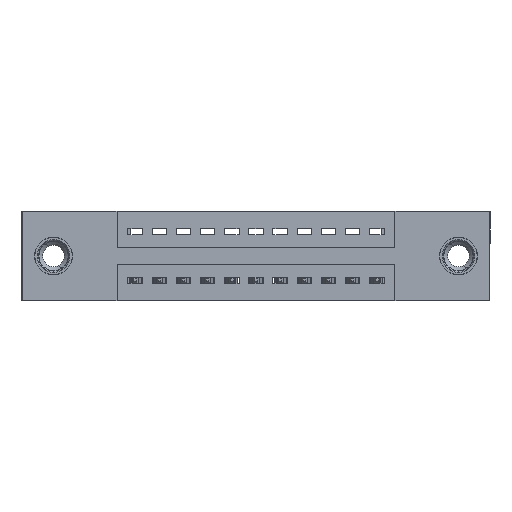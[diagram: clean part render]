
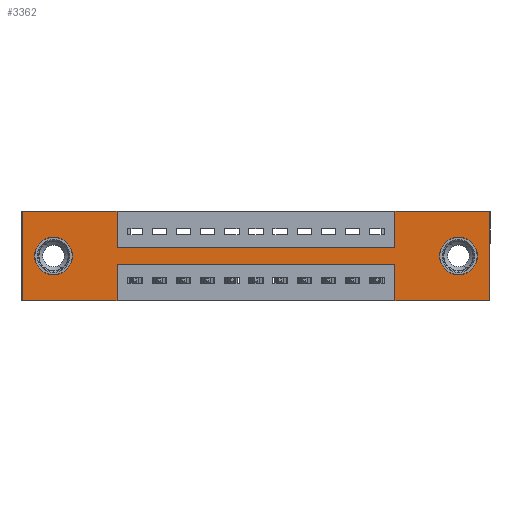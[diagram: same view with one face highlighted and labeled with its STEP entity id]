
A CAD part, front view. The second image highlights one B-rep face of the part: STEP entity #3362.
In plain terms, the highlighted planar face has unit normal (0, -1, 0).
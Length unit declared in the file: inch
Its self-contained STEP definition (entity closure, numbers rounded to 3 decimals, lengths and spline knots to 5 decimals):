
#35 = CARTESIAN_POINT ( 'NONE',  ( 0.3925, 0., -0.22 ) ) ;
#104 = ORIENTED_EDGE ( 'NONE', *, *, #4756, .T. ) ;
#218 = EDGE_LOOP ( 'NONE', ( #4142, #5521, #10170, #14309, #9208, #8165, #9897, #368, #8636, #7053, #12639, #8810 ) ) ;
#368 = ORIENTED_EDGE ( 'NONE', *, *, #10709, .F. ) ;
#396 = EDGE_CURVE ( 'NONE', #11359, #4850, #6429, .T. ) ;
#531 = DIRECTION ( 'NONE',  ( 0., 1., 0. ) ) ;
#616 = ORIENTED_EDGE ( 'NONE', *, *, #11201, .T. ) ;
#686 = CARTESIAN_POINT ( 'NONE',  ( 0., 0., 0. ) ) ;
#900 = CARTESIAN_POINT ( 'NONE',  ( 0.3925, 0., -0.22 ) ) ;
#925 = CIRCLE ( 'NONE', #3163, 0.078 ) ;
#931 = DIRECTION ( 'NONE',  ( 0., 0., -1. ) ) ;
#985 = EDGE_CURVE ( 'NONE', #6695, #3513, #13097, .T. ) ;
#1330 = CARTESIAN_POINT ( 'NONE',  ( 1.5425, 0., -0.37 ) ) ;
#1398 = DIRECTION ( 'NONE',  ( 0., 0., -1. ) ) ;
#1551 = VECTOR ( 'NONE', #5453, 39.37008 ) ;
#1705 = LINE ( 'NONE', #4339, #5451 ) ;
#2826 = CARTESIAN_POINT ( 'NONE',  ( 1.5425, 0., 0. ) ) ;
#2831 = CARTESIAN_POINT ( 'NONE',  ( 1.5425, 0., 0. ) ) ;
#3046 = VECTOR ( 'NONE', #9522, 39.37008 ) ;
#3136 = ORIENTED_EDGE ( 'NONE', *, *, #4229, .T. ) ;
#3163 = AXIS2_PLACEMENT_3D ( 'NONE', #7218, #8627, #7538 ) ;
#3184 = CARTESIAN_POINT ( 'NONE',  ( 0., 0., -0.37 ) ) ;
#3260 = FACE_BOUND ( 'NONE', #8685, .T. ) ;
#3316 = VECTOR ( 'NONE', #7759, 39.37008 ) ;
#3362 = ADVANCED_FACE ( 'NONE', ( #3260, #12242, #5032 ), #12625, .T. ) ;
#3400 = VERTEX_POINT ( 'NONE', #4562 ) ;
#3513 = VERTEX_POINT ( 'NONE', #10838 ) ;
#3675 = LINE ( 'NONE', #1330, #3316 ) ;
#3700 = VERTEX_POINT ( 'NONE', #14413 ) ;
#4052 = VERTEX_POINT ( 'NONE', #11518 ) ;
#4142 = ORIENTED_EDGE ( 'NONE', *, *, #396, .F. ) ;
#4229 = EDGE_CURVE ( 'NONE', #8845, #3400, #925, .T. ) ;
#4248 = EDGE_CURVE ( 'NONE', #3700, #9890, #11864, .T. ) ;
#4339 = CARTESIAN_POINT ( 'NONE',  ( 0., 0., -0.37 ) ) ;
#4347 = LINE ( 'NONE', #686, #11399 ) ;
#4562 = CARTESIAN_POINT ( 'NONE',  ( 0.13, 0., -0.263 ) ) ;
#4598 = LINE ( 'NONE', #2831, #3046 ) ;
#4756 = EDGE_CURVE ( 'NONE', #3513, #6695, #10090, .T. ) ;
#4850 = VERTEX_POINT ( 'NONE', #12964 ) ;
#5030 = AXIS2_PLACEMENT_3D ( 'NONE', #9568, #531, #9363 ) ;
#5032 = FACE_OUTER_BOUND ( 'NONE', #218, .T. ) ;
#5337 = CARTESIAN_POINT ( 'NONE',  ( 0.3925, 0., 0. ) ) ;
#5451 = VECTOR ( 'NONE', #7333, 39.37008 ) ;
#5453 = DIRECTION ( 'NONE',  ( -1., 0., 0. ) ) ;
#5521 = ORIENTED_EDGE ( 'NONE', *, *, #5659, .F. ) ;
#5659 = EDGE_CURVE ( 'NONE', #7968, #11359, #7574, .T. ) ;
#5713 = CARTESIAN_POINT ( 'NONE',  ( 0., 0., 0. ) ) ;
#5814 = VERTEX_POINT ( 'NONE', #6860 ) ;
#5987 = VERTEX_POINT ( 'NONE', #8358 ) ;
#5991 = DIRECTION ( 'NONE',  ( 0., 1., 0. ) ) ;
#6126 = VERTEX_POINT ( 'NONE', #2826 ) ;
#6256 = DIRECTION ( 'NONE',  ( 0., 0., -1. ) ) ;
#6429 = LINE ( 'NONE', #11588, #11881 ) ;
#6695 = VERTEX_POINT ( 'NONE', #10390 ) ;
#6750 = VECTOR ( 'NONE', #931, 39.37008 ) ;
#6860 = CARTESIAN_POINT ( 'NONE',  ( 1.935, 0., 0. ) ) ;
#6983 = CARTESIAN_POINT ( 'NONE',  ( 0., 0., -0.37 ) ) ;
#7030 = EDGE_CURVE ( 'NONE', #5814, #4052, #7908, .T. ) ;
#7053 = ORIENTED_EDGE ( 'NONE', *, *, #8544, .F. ) ;
#7171 = VECTOR ( 'NONE', #10931, 39.37008 ) ;
#7202 = DIRECTION ( 'NONE',  ( 1., 0., 0. ) ) ;
#7218 = CARTESIAN_POINT ( 'NONE',  ( 0.13, 0., -0.185 ) ) ;
#7333 = DIRECTION ( 'NONE',  ( -1., 0., 0. ) ) ;
#7452 = CARTESIAN_POINT ( 'NONE',  ( 0., 0., 0. ) ) ;
#7538 = DIRECTION ( 'NONE',  ( 0., 0., 1. ) ) ;
#7574 = LINE ( 'NONE', #900, #1551 ) ;
#7759 = DIRECTION ( 'NONE',  ( 0., 0., 1. ) ) ;
#7908 = LINE ( 'NONE', #12258, #11277 ) ;
#7968 = VERTEX_POINT ( 'NONE', #9974 ) ;
#7976 = EDGE_CURVE ( 'NONE', #4850, #5987, #10179, .T. ) ;
#8165 = ORIENTED_EDGE ( 'NONE', *, *, #10068, .F. ) ;
#8335 = LINE ( 'NONE', #13434, #10112 ) ;
#8358 = CARTESIAN_POINT ( 'NONE',  ( 0., 0., -0.37 ) ) ;
#8544 = EDGE_CURVE ( 'NONE', #9881, #3700, #4347, .T. ) ;
#8560 = CARTESIAN_POINT ( 'NONE',  ( 0.13, 0., -0.107 ) ) ;
#8627 = DIRECTION ( 'NONE',  ( 0., 1., 0. ) ) ;
#8636 = ORIENTED_EDGE ( 'NONE', *, *, #4248, .F. ) ;
#8667 = CIRCLE ( 'NONE', #5030, 0.078 ) ;
#8685 = EDGE_LOOP ( 'NONE', ( #10910, #104 ) ) ;
#8810 = ORIENTED_EDGE ( 'NONE', *, *, #7976, .F. ) ;
#8845 = VERTEX_POINT ( 'NONE', #8560 ) ;
#8944 = VERTEX_POINT ( 'NONE', #10645 ) ;
#9088 = AXIS2_PLACEMENT_3D ( 'NONE', #12718, #5991, #10472 ) ;
#9128 = DIRECTION ( 'NONE',  ( 0., 0., 1. ) ) ;
#9208 = ORIENTED_EDGE ( 'NONE', *, *, #7030, .F. ) ;
#9355 = CARTESIAN_POINT ( 'NONE',  ( 0.3925, 0., -0.15 ) ) ;
#9363 = DIRECTION ( 'NONE',  ( 0., 0., 1. ) ) ;
#9522 = DIRECTION ( 'NONE',  ( 0., 0., 1. ) ) ;
#9568 = CARTESIAN_POINT ( 'NONE',  ( 0.13, 0., -0.185 ) ) ;
#9624 = CARTESIAN_POINT ( 'NONE',  ( 1.805, 0., -0.185 ) ) ;
#9800 = VECTOR ( 'NONE', #9128, 39.37008 ) ;
#9881 = VERTEX_POINT ( 'NONE', #7452 ) ;
#9890 = VERTEX_POINT ( 'NONE', #12040 ) ;
#9897 = ORIENTED_EDGE ( 'NONE', *, *, #11224, .F. ) ;
#9904 = DIRECTION ( 'NONE',  ( 1., 0., 0. ) ) ;
#9974 = CARTESIAN_POINT ( 'NONE',  ( 1.5425, 0., -0.22 ) ) ;
#10068 = EDGE_CURVE ( 'NONE', #6126, #5814, #8335, .T. ) ;
#10090 = CIRCLE ( 'NONE', #9088, 0.078 ) ;
#10112 = VECTOR ( 'NONE', #12706, 39.37008 ) ;
#10170 = ORIENTED_EDGE ( 'NONE', *, *, #13277, .F. ) ;
#10179 = LINE ( 'NONE', #3184, #7171 ) ;
#10390 = CARTESIAN_POINT ( 'NONE',  ( 1.805, 0., -0.107 ) ) ;
#10472 = DIRECTION ( 'NONE',  ( 0., 0., -1. ) ) ;
#10645 = CARTESIAN_POINT ( 'NONE',  ( 1.5425, 0., -0.15 ) ) ;
#10709 = EDGE_CURVE ( 'NONE', #9890, #8944, #12711, .T. ) ;
#10838 = CARTESIAN_POINT ( 'NONE',  ( 1.805, 0., -0.263 ) ) ;
#10910 = ORIENTED_EDGE ( 'NONE', *, *, #985, .T. ) ;
#10931 = DIRECTION ( 'NONE',  ( -1., 0., 0. ) ) ;
#11110 = EDGE_LOOP ( 'NONE', ( #3136, #616 ) ) ;
#11154 = VECTOR ( 'NONE', #7202, 39.37008 ) ;
#11201 = EDGE_CURVE ( 'NONE', #3400, #8845, #8667, .T. ) ;
#11224 = EDGE_CURVE ( 'NONE', #8944, #6126, #4598, .T. ) ;
#11239 = VERTEX_POINT ( 'NONE', #12968 ) ;
#11277 = VECTOR ( 'NONE', #11570, 39.37008 ) ;
#11359 = VERTEX_POINT ( 'NONE', #35 ) ;
#11399 = VECTOR ( 'NONE', #9904, 39.37008 ) ;
#11518 = CARTESIAN_POINT ( 'NONE',  ( 1.935, 0., -0.37 ) ) ;
#11523 = DIRECTION ( 'NONE',  ( 0., -1., 0. ) ) ;
#11570 = DIRECTION ( 'NONE',  ( 0., 0., -1. ) ) ;
#11588 = CARTESIAN_POINT ( 'NONE',  ( 0.3925, 0., -0.37 ) ) ;
#11864 = LINE ( 'NONE', #5337, #6750 ) ;
#11881 = VECTOR ( 'NONE', #1398, 39.37008 ) ;
#12040 = CARTESIAN_POINT ( 'NONE',  ( 0.3925, 0., -0.15 ) ) ;
#12242 = FACE_BOUND ( 'NONE', #11110, .T. ) ;
#12258 = CARTESIAN_POINT ( 'NONE',  ( 1.935, 0., 0. ) ) ;
#12483 = EDGE_CURVE ( 'NONE', #4052, #11239, #1705, .T. ) ;
#12625 = PLANE ( 'NONE',  #14304 ) ;
#12639 = ORIENTED_EDGE ( 'NONE', *, *, #14211, .F. ) ;
#12706 = DIRECTION ( 'NONE',  ( 1., 0., 0. ) ) ;
#12711 = LINE ( 'NONE', #9355, #11154 ) ;
#12718 = CARTESIAN_POINT ( 'NONE',  ( 1.805, 0., -0.185 ) ) ;
#12964 = CARTESIAN_POINT ( 'NONE',  ( 0.3925, 0., -0.37 ) ) ;
#12968 = CARTESIAN_POINT ( 'NONE',  ( 1.5425, 0., -0.37 ) ) ;
#12981 = DIRECTION ( 'NONE',  ( 0., 1., 0. ) ) ;
#13097 = CIRCLE ( 'NONE', #13497, 0.078 ) ;
#13277 = EDGE_CURVE ( 'NONE', #11239, #7968, #3675, .T. ) ;
#13434 = CARTESIAN_POINT ( 'NONE',  ( 0., 0., 0. ) ) ;
#13497 = AXIS2_PLACEMENT_3D ( 'NONE', #9624, #12981, #6256 ) ;
#13696 = DIRECTION ( 'NONE',  ( 0., 0., -1. ) ) ;
#14211 = EDGE_CURVE ( 'NONE', #5987, #9881, #14376, .T. ) ;
#14304 = AXIS2_PLACEMENT_3D ( 'NONE', #6983, #11523, #13696 ) ;
#14309 = ORIENTED_EDGE ( 'NONE', *, *, #12483, .F. ) ;
#14376 = LINE ( 'NONE', #5713, #9800 ) ;
#14413 = CARTESIAN_POINT ( 'NONE',  ( 0.3925, 0., 0. ) ) ;
